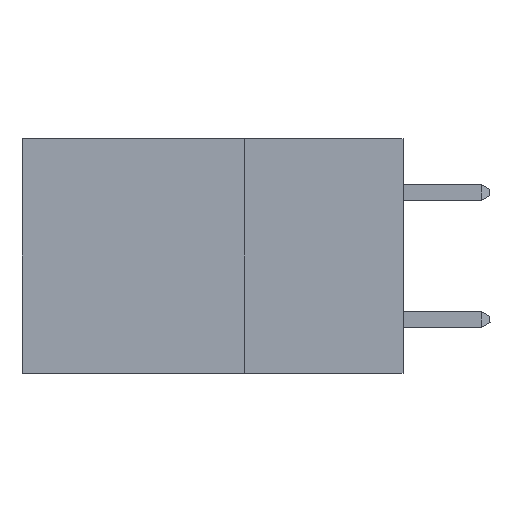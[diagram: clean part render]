
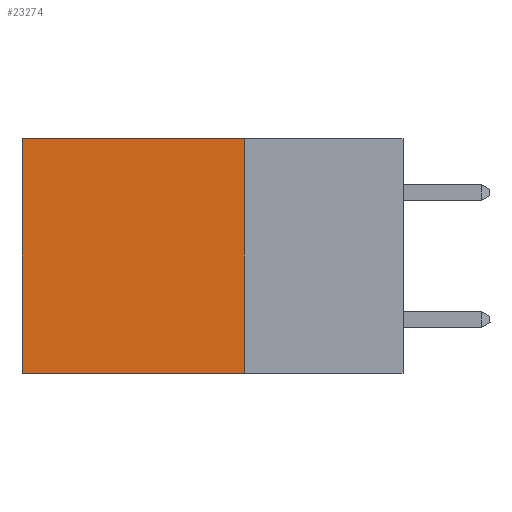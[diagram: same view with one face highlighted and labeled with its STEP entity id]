
A CAD part, left-side view. The second image highlights one B-rep face of the part: STEP entity #23274.
In plain terms, the highlighted planar face has unit normal (-1, 0, 0).
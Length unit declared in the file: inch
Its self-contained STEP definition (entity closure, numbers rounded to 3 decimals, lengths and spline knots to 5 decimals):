
#365 = ORIENTED_EDGE ( 'NONE', *, *, #6510, .F. ) ;
#1889 = VECTOR ( 'NONE', #28238, 39.37008 ) ;
#3187 = FACE_OUTER_BOUND ( 'NONE', #16818, .T. ) ;
#4331 = EDGE_CURVE ( 'NONE', #12767, #18801, #38830, .T. ) ;
#4354 = EDGE_CURVE ( 'NONE', #18801, #23588, #24370, .T. ) ;
#5081 = DIRECTION ( 'NONE',  ( 0., 0., -1. ) ) ;
#6349 = VECTOR ( 'NONE', #19193, 39.37008 ) ;
#6510 = EDGE_CURVE ( 'NONE', #15898, #23588, #36164, .T. ) ;
#9013 = ORIENTED_EDGE ( 'NONE', *, *, #36958, .F. ) ;
#11857 = PLANE ( 'NONE',  #37790 ) ;
#12510 = CARTESIAN_POINT ( 'NONE',  ( 0.2875, 0.6, 0. ) ) ;
#12767 = VERTEX_POINT ( 'NONE', #20647 ) ;
#15898 = VERTEX_POINT ( 'NONE', #41077 ) ;
#16818 = EDGE_LOOP ( 'NONE', ( #22583, #365, #9013, #37025 ) ) ;
#18066 = CARTESIAN_POINT ( 'NONE',  ( 0.2875, 0.25, 0. ) ) ;
#18555 = DIRECTION ( 'NONE',  ( 1., 0., 0. ) ) ;
#18801 = VERTEX_POINT ( 'NONE', #37437 ) ;
#19193 = DIRECTION ( 'NONE',  ( 0., 1., 0. ) ) ;
#20647 = CARTESIAN_POINT ( 'NONE',  ( 0.2875, 0.25, 0. ) ) ;
#22435 = DIRECTION ( 'NONE',  ( 0., 1., 0. ) ) ;
#22583 = ORIENTED_EDGE ( 'NONE', *, *, #4354, .T. ) ;
#23274 = ADVANCED_FACE ( 'NONE', ( #3187 ), #11857, .F. ) ;
#23588 = VERTEX_POINT ( 'NONE', #35378 ) ;
#24370 = LINE ( 'NONE', #12510, #1889 ) ;
#28238 = DIRECTION ( 'NONE',  ( 0., 0., -1. ) ) ;
#28679 = VECTOR ( 'NONE', #5081, 39.37008 ) ;
#28697 = VECTOR ( 'NONE', #22435, 39.37008 ) ;
#30677 = LINE ( 'NONE', #18066, #28679 ) ;
#31556 = CARTESIAN_POINT ( 'NONE',  ( 0.2875, 0.25, 0. ) ) ;
#34422 = CARTESIAN_POINT ( 'NONE',  ( 0.2875, 0.25, 0. ) ) ;
#35378 = CARTESIAN_POINT ( 'NONE',  ( 0.2875, 0.6, -0.37 ) ) ;
#36164 = LINE ( 'NONE', #40232, #28697 ) ;
#36958 = EDGE_CURVE ( 'NONE', #12767, #15898, #30677, .T. ) ;
#37025 = ORIENTED_EDGE ( 'NONE', *, *, #4331, .T. ) ;
#37215 = DIRECTION ( 'NONE',  ( 0., 0., -1. ) ) ;
#37437 = CARTESIAN_POINT ( 'NONE',  ( 0.2875, 0.6, 0. ) ) ;
#37790 = AXIS2_PLACEMENT_3D ( 'NONE', #34422, #18555, #37215 ) ;
#38830 = LINE ( 'NONE', #31556, #6349 ) ;
#40232 = CARTESIAN_POINT ( 'NONE',  ( 0.2875, 0.25, -0.37 ) ) ;
#41077 = CARTESIAN_POINT ( 'NONE',  ( 0.2875, 0.25, -0.37 ) ) ;
